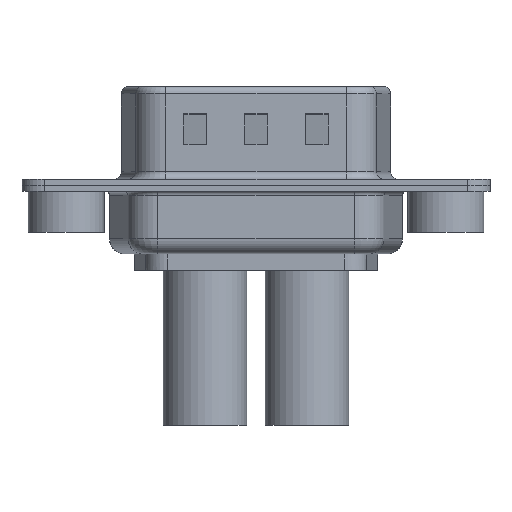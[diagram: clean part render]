
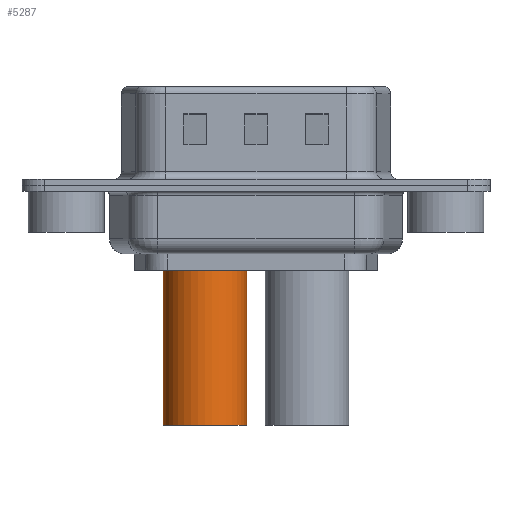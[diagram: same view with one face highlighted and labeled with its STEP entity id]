
A CAD part, front view. The second image highlights one B-rep face of the part: STEP entity #5287.
In plain terms, the highlighted cylindrical face has radius 2.75 mm (diameter 5.5 mm), a partial arc.
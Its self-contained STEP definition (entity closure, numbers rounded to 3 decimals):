
#154 = ORIENTED_EDGE ( 'NONE', *, *, #11436, .T. ) ;
#428 = DIRECTION ( 'NONE',  ( 0., 0., -1. ) ) ;
#879 = ORIENTED_EDGE ( 'NONE', *, *, #7801, .T. ) ;
#1545 = EDGE_CURVE ( 'NONE', #11063, #5317, #2697, .T. ) ;
#1683 = VECTOR ( 'NONE', #428, 1000. ) ;
#1842 = VERTEX_POINT ( 'NONE', #4348 ) ;
#1985 = EDGE_LOOP ( 'NONE', ( #8563, #154, #12688, #9767, #879, #5875 ) ) ;
#2559 = CARTESIAN_POINT ( 'NONE',  ( -2.75, 0., -7.764 ) ) ;
#2637 = CARTESIAN_POINT ( 'NONE',  ( 0., 0., 4.234 ) ) ;
#2697 = CIRCLE ( 'NONE', #8434, 2.75 ) ;
#3365 = DIRECTION ( 'NONE',  ( 0., 0., 1. ) ) ;
#4055 = LINE ( 'NONE', #13165, #9702 ) ;
#4137 = VERTEX_POINT ( 'NONE', #6183 ) ;
#4198 = VERTEX_POINT ( 'NONE', #9374 ) ;
#4348 = CARTESIAN_POINT ( 'NONE',  ( 2.75, 0., -8.7 ) ) ;
#4476 = DIRECTION ( 'NONE',  ( 0., 0., 1. ) ) ;
#4511 = CARTESIAN_POINT ( 'NONE',  ( 2.75, 0., 1.5 ) ) ;
#4614 = AXIS2_PLACEMENT_3D ( 'NONE', #8767, #8740, #8659 ) ;
#4748 = EDGE_CURVE ( 'NONE', #4198, #1842, #8258, .T. ) ;
#4821 = CARTESIAN_POINT ( 'NONE',  ( 2.75, 0., -8.7 ) ) ;
#5244 = CYLINDRICAL_SURFACE ( 'NONE', #11038, 2.75 ) ;
#5287 = ADVANCED_FACE ( 'NONE', ( #8576 ), #5244, .T. ) ;
#5317 = VERTEX_POINT ( 'NONE', #4511 ) ;
#5693 = CARTESIAN_POINT ( 'NONE',  ( 2.75, 0., 4.234 ) ) ;
#5875 = ORIENTED_EDGE ( 'NONE', *, *, #1545, .F. ) ;
#6183 = CARTESIAN_POINT ( 'NONE',  ( -2.75, 0., -8.7 ) ) ;
#6284 = DIRECTION ( 'NONE',  ( 0., 0., 1. ) ) ;
#6564 = EDGE_CURVE ( 'NONE', #13017, #11063, #14423, .T. ) ;
#7092 = EDGE_CURVE ( 'NONE', #4137, #1842, #10396, .T. ) ;
#7801 = EDGE_CURVE ( 'NONE', #4198, #5317, #13240, .T. ) ;
#8205 = CARTESIAN_POINT ( 'NONE',  ( -2.75, 0., 1.5 ) ) ;
#8258 = LINE ( 'NONE', #4821, #1683 ) ;
#8377 = VECTOR ( 'NONE', #10333, 1000. ) ;
#8434 = AXIS2_PLACEMENT_3D ( 'NONE', #9115, #6284, #9146 ) ;
#8563 = ORIENTED_EDGE ( 'NONE', *, *, #6564, .F. ) ;
#8576 = FACE_OUTER_BOUND ( 'NONE', #1985, .T. ) ;
#8659 = DIRECTION ( 'NONE',  ( 1., 0., 0. ) ) ;
#8740 = DIRECTION ( 'NONE',  ( 0., 0., 1. ) ) ;
#8767 = CARTESIAN_POINT ( 'NONE',  ( 0., 0., -8.7 ) ) ;
#9115 = CARTESIAN_POINT ( 'NONE',  ( 0., 0., 1.5 ) ) ;
#9146 = DIRECTION ( 'NONE',  ( 1., 0., 0. ) ) ;
#9374 = CARTESIAN_POINT ( 'NONE',  ( 2.75, 0., -7.764 ) ) ;
#9702 = VECTOR ( 'NONE', #12099, 1000. ) ;
#9767 = ORIENTED_EDGE ( 'NONE', *, *, #4748, .F. ) ;
#10227 = CARTESIAN_POINT ( 'NONE',  ( -2.75, 0., 4.234 ) ) ;
#10333 = DIRECTION ( 'NONE',  ( 0., 0., 1. ) ) ;
#10396 = CIRCLE ( 'NONE', #4614, 2.75 ) ;
#11038 = AXIS2_PLACEMENT_3D ( 'NONE', #2637, #3365, #11913 ) ;
#11063 = VERTEX_POINT ( 'NONE', #8205 ) ;
#11436 = EDGE_CURVE ( 'NONE', #13017, #4137, #4055, .T. ) ;
#11897 = VECTOR ( 'NONE', #4476, 1000. ) ;
#11913 = DIRECTION ( 'NONE',  ( 1., 0., 0. ) ) ;
#12099 = DIRECTION ( 'NONE',  ( 0., 0., -1. ) ) ;
#12688 = ORIENTED_EDGE ( 'NONE', *, *, #7092, .T. ) ;
#13017 = VERTEX_POINT ( 'NONE', #2559 ) ;
#13165 = CARTESIAN_POINT ( 'NONE',  ( -2.75, 0., -8.7 ) ) ;
#13240 = LINE ( 'NONE', #5693, #11897 ) ;
#14423 = LINE ( 'NONE', #10227, #8377 ) ;
